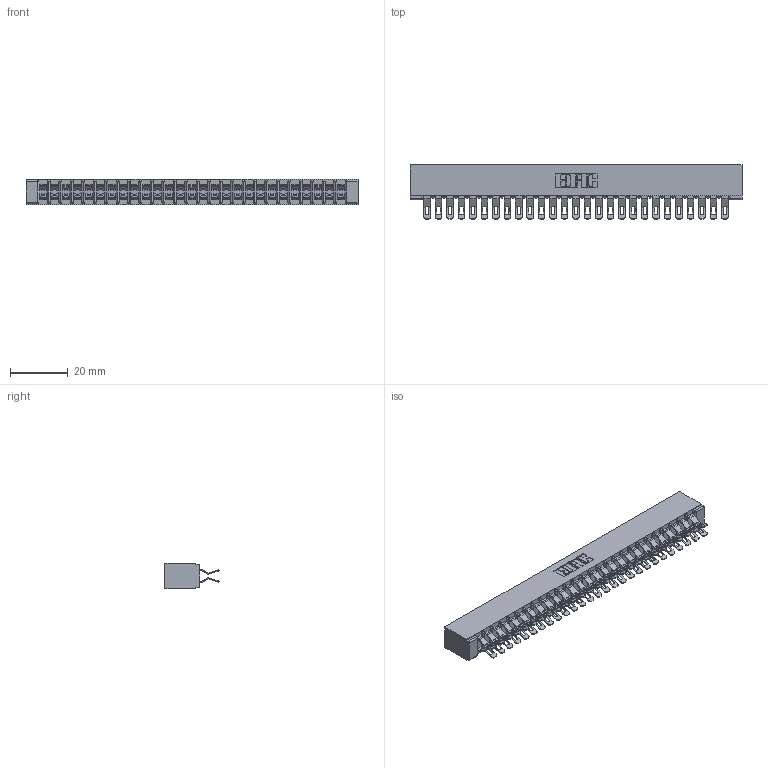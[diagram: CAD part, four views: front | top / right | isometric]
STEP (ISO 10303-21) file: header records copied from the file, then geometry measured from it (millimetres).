
FILE_DESCRIPTION (( 'STEP AP203' ), '1' );
FILE_NAME ('357-054-455-201.STEP', '2020-10-04T08:52:20', ( '' ), ( '' ), 'SwSTEP 2.0', 'SolidWorks 2020', '' );
FILE_SCHEMA (( 'CONFIG_CONTROL_DESIGN' ));
Length unit declared in the file: inch
Products named in the file (3): 307-290-001_555; 357-054-455-201; 307 Part_No Mounting Lugs
Assembly tree (55 placements, depth 2):
  357-054-455-201
    307 Part_No Mounting Lugs
    307-290-001_555  x54
Bounding box: 114.86 x 18.75 x 8.71 mm (x, y, z)
Volume: 7906.4 mm3; surface area: 15584.7 mm2
Topology: 55 solids, 55 shells, 3432 faces, 10073 edges, 6566 vertices
Faces by surface type: plane 1902, cylinder 1474, sphere 56
Entity records: 26119 total; most frequent: CARTESIAN_POINT 4279, ORIENTED_EDGE 4240, DIRECTION 4204, EDGE_CURVE 2120, LINE 1610, VECTOR 1610, VERTEX_POINT 1372, AXIS2_PLACEMENT_3D 1297
